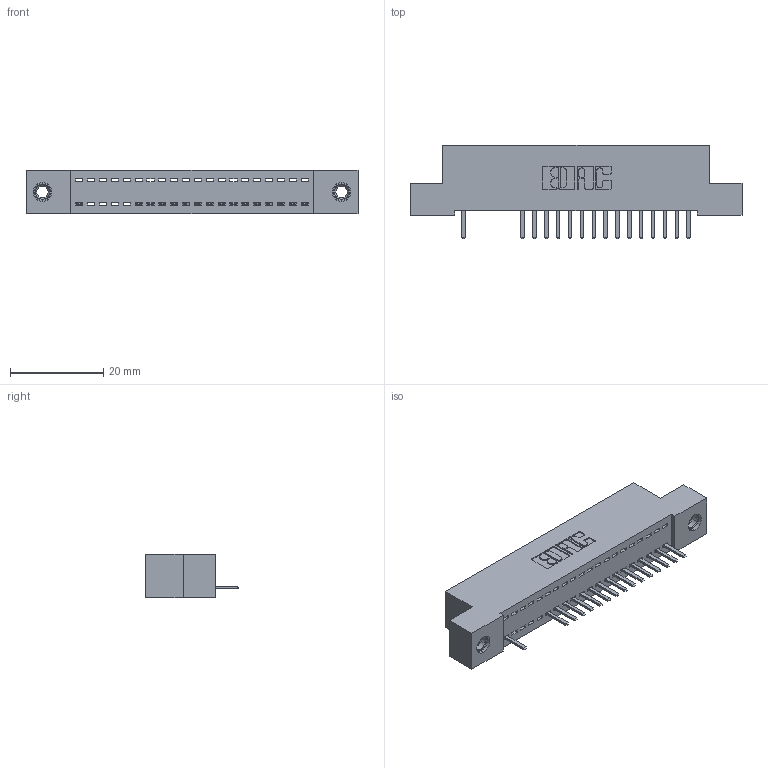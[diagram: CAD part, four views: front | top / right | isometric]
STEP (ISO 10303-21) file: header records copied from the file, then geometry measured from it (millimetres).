
FILE_DESCRIPTION (( 'STEP AP203' ), '1' );
FILE_NAME ('392-020-520-107.STEP', '2018-08-15T05:51:55', ( '' ), ( '' ), 'SwSTEP 2.0', 'SolidWorks 2016', '' );
FILE_SCHEMA (( 'CONFIG_CONTROL_DESIGN' ));
Length unit declared in the file: inch
Products named in the file (4): 342 Part_TI; 345-292-001_345-293-120; 345-250-001_345-250-005-103; 392-020-520-107
Assembly tree (19 placements, depth 2):
  392-020-520-107
    342 Part_TI
    345-292-001_345-293-120  x16
    345-250-001_345-250-005-103  x2
Bounding box: 71.12 x 20.02 x 9.4 mm (x, y, z)
Volume: 6050.3 mm3; surface area: 8121.8 mm2
Topology: 19 solids, 19 shells, 1210 faces, 3547 edges, 2314 vertices
Faces by surface type: plane 850, cylinder 344, cone 12, torus 4
Entity records: 16112 total; most frequent: CARTESIAN_POINT 2793, ORIENTED_EDGE 2734, DIRECTION 2417, EDGE_CURVE 1367, LINE 1215, VECTOR 1215, VERTEX_POINT 904, AXIS2_PLACEMENT_3D 601
